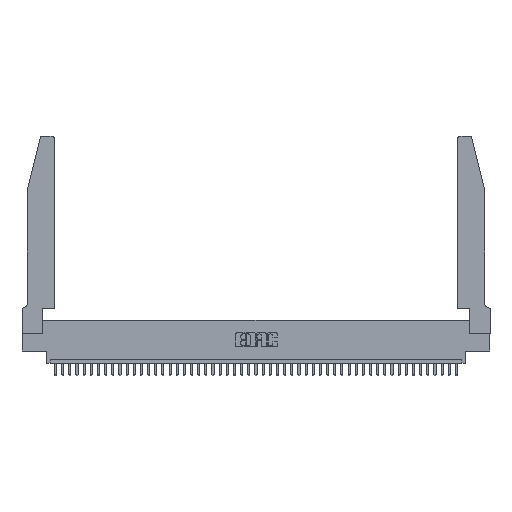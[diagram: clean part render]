
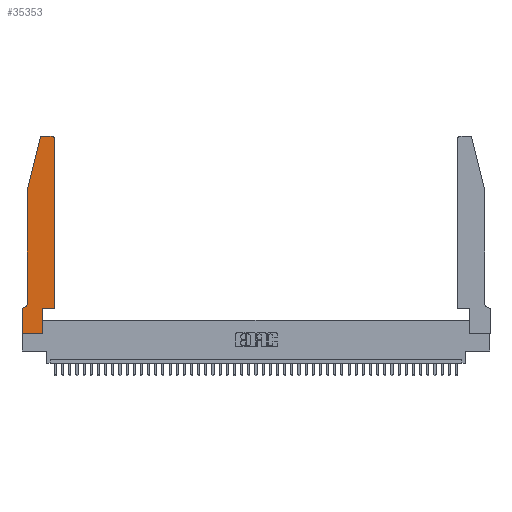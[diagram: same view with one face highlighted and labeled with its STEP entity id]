
A CAD part, top view. The second image highlights one B-rep face of the part: STEP entity #35353.
In plain terms, the highlighted planar face has unit normal (0, 0, 1).
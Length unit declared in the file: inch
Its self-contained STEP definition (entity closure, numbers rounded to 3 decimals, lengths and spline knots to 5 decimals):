
#238 = ORIENTED_EDGE ( 'NONE', *, *, #34138, .T. ) ;
#360 = EDGE_CURVE ( 'NONE', #20974, #18278, #41906, .T. ) ;
#923 = CARTESIAN_POINT ( 'NONE',  ( 0., 0.35, 0.37 ) ) ;
#1006 = CARTESIAN_POINT ( 'NONE',  ( 0., 0., 0.37 ) ) ;
#1175 = CARTESIAN_POINT ( 'NONE',  ( 0.2605, 2.75, 0.37 ) ) ;
#1420 = CARTESIAN_POINT ( 'NONE',  ( 0.2865, 0.35, 0.37 ) ) ;
#1841 = DIRECTION ( 'NONE',  ( 1., 0., 0. ) ) ;
#2367 = ORIENTED_EDGE ( 'NONE', *, *, #9281, .T. ) ;
#2576 = ORIENTED_EDGE ( 'NONE', *, *, #35961, .T. ) ;
#2604 = LINE ( 'NONE', #16483, #27012 ) ;
#2642 = CARTESIAN_POINT ( 'NONE',  ( 0.2865, 0.35, 0.37 ) ) ;
#3133 = DIRECTION ( 'NONE',  ( -1., 0., 0. ) ) ;
#3793 = ORIENTED_EDGE ( 'NONE', *, *, #360, .T. ) ;
#4416 = CARTESIAN_POINT ( 'NONE',  ( 0., 0.35, 0.37 ) ) ;
#4430 = DIRECTION ( 'NONE',  ( -1., 0., 0. ) ) ;
#4469 = ORIENTED_EDGE ( 'NONE', *, *, #27929, .T. ) ;
#4613 = CARTESIAN_POINT ( 'NONE',  ( 0., 0., 0.37 ) ) ;
#4697 = CARTESIAN_POINT ( 'NONE',  ( 0.4505, 0.35, 0.37 ) ) ;
#5005 = VECTOR ( 'NONE', #39588, 39.37008 ) ;
#5119 = CARTESIAN_POINT ( 'NONE',  ( 0.0755, 2., 0.37 ) ) ;
#5654 = CIRCLE ( 'NONE', #28193, 0.07 ) ;
#6397 = VERTEX_POINT ( 'NONE', #923 ) ;
#6874 = CARTESIAN_POINT ( 'NONE',  ( 0.2865, 0., 0.37 ) ) ;
#7835 = DIRECTION ( 'NONE',  ( 1., 0., 0. ) ) ;
#7964 = CARTESIAN_POINT ( 'NONE',  ( 0.0755, 2., 0.37 ) ) ;
#8586 = CARTESIAN_POINT ( 'NONE',  ( 0.4505, 0.35, 0.37 ) ) ;
#8760 = DIRECTION ( 'NONE',  ( 0., -1., 0. ) ) ;
#8840 = VECTOR ( 'NONE', #31406, 39.37008 ) ;
#9281 = EDGE_CURVE ( 'NONE', #23190, #41723, #2604, .T. ) ;
#10288 = ORIENTED_EDGE ( 'NONE', *, *, #40681, .T. ) ;
#10289 = DIRECTION ( 'NONE',  ( 0., 0., -1. ) ) ;
#10429 = CARTESIAN_POINT ( 'NONE',  ( 0.0055, 0.35, 0.37 ) ) ;
#10708 = EDGE_CURVE ( 'NONE', #18545, #32068, #42664, .T. ) ;
#10870 = EDGE_LOOP ( 'NONE', ( #25794, #3793, #2576, #2367, #238, #40316, #20982, #4469, #16432, #30273, #12661, #10288 ) ) ;
#10888 = EDGE_CURVE ( 'NONE', #21116, #18545, #12234, .T. ) ;
#11809 = DIRECTION ( 'NONE',  ( -0.239, -0.971, 0. ) ) ;
#11862 = PLANE ( 'NONE',  #31098 ) ;
#12083 = VECTOR ( 'NONE', #36885, 39.37008 ) ;
#12234 = LINE ( 'NONE', #1420, #22256 ) ;
#12385 = DIRECTION ( 'NONE',  ( 1., 0., 0. ) ) ;
#12661 = ORIENTED_EDGE ( 'NONE', *, *, #30907, .T. ) ;
#13523 = CARTESIAN_POINT ( 'NONE',  ( 0.0055, 0.42, 0.37 ) ) ;
#15779 = DIRECTION ( 'NONE',  ( 0., 0., 1. ) ) ;
#16129 = LINE ( 'NONE', #1175, #27207 ) ;
#16432 = ORIENTED_EDGE ( 'NONE', *, *, #10888, .T. ) ;
#16483 = CARTESIAN_POINT ( 'NONE',  ( 0.0755, 2., 0.37 ) ) ;
#16660 = LINE ( 'NONE', #1006, #5005 ) ;
#16927 = EDGE_CURVE ( 'NONE', #45058, #6397, #34087, .T. ) ;
#17163 = LINE ( 'NONE', #8586, #8840 ) ;
#18278 = VERTEX_POINT ( 'NONE', #44813 ) ;
#18534 = DIRECTION ( 'NONE',  ( 0., 0., 1. ) ) ;
#18545 = VERTEX_POINT ( 'NONE', #2642 ) ;
#20974 = VERTEX_POINT ( 'NONE', #28274 ) ;
#20982 = ORIENTED_EDGE ( 'NONE', *, *, #26684, .T. ) ;
#21116 = VERTEX_POINT ( 'NONE', #6874 ) ;
#22256 = VECTOR ( 'NONE', #33385, 39.37008 ) ;
#23190 = VERTEX_POINT ( 'NONE', #7964 ) ;
#23413 = AXIS2_PLACEMENT_3D ( 'NONE', #28247, #35282, #38821 ) ;
#24199 = CARTESIAN_POINT ( 'NONE',  ( 0.0755, 0.35, 0.37 ) ) ;
#25794 = ORIENTED_EDGE ( 'NONE', *, *, #38031, .T. ) ;
#26684 = EDGE_CURVE ( 'NONE', #6397, #29456, #16660, .T. ) ;
#27012 = VECTOR ( 'NONE', #8760, 39.37008 ) ;
#27207 = VECTOR ( 'NONE', #4430, 39.37008 ) ;
#27929 = EDGE_CURVE ( 'NONE', #29456, #21116, #40213, .T. ) ;
#28193 = AXIS2_PLACEMENT_3D ( 'NONE', #13523, #10289, #3133 ) ;
#28247 = CARTESIAN_POINT ( 'NONE',  ( 0.284, 2.72, 0.37 ) ) ;
#28274 = CARTESIAN_POINT ( 'NONE',  ( 0.284, 2.75, 0.37 ) ) ;
#28393 = CARTESIAN_POINT ( 'NONE',  ( 0.4505, 2.72, 0.37 ) ) ;
#29456 = VERTEX_POINT ( 'NONE', #43304 ) ;
#29823 = CARTESIAN_POINT ( 'NONE',  ( 0.4505, 0.35, 0.37 ) ) ;
#30273 = ORIENTED_EDGE ( 'NONE', *, *, #10708, .T. ) ;
#30513 = VERTEX_POINT ( 'NONE', #28393 ) ;
#30907 = EDGE_CURVE ( 'NONE', #32068, #30513, #17163, .T. ) ;
#31098 = AXIS2_PLACEMENT_3D ( 'NONE', #4416, #18534, #7835 ) ;
#31406 = DIRECTION ( 'NONE',  ( 0., 1., 0. ) ) ;
#32068 = VERTEX_POINT ( 'NONE', #4697 ) ;
#33385 = DIRECTION ( 'NONE',  ( 0., 1., 0. ) ) ;
#33811 = CIRCLE ( 'NONE', #43741, 0.03 ) ;
#34087 = LINE ( 'NONE', #24199, #39618 ) ;
#34138 = EDGE_CURVE ( 'NONE', #41723, #45058, #5654, .T. ) ;
#34336 = VECTOR ( 'NONE', #12385, 39.37008 ) ;
#35140 = DIRECTION ( 'NONE',  ( -1., 0., 0. ) ) ;
#35282 = DIRECTION ( 'NONE',  ( 0., 0., 1. ) ) ;
#35353 = ADVANCED_FACE ( 'NONE', ( #40342 ), #11862, .T. ) ;
#35558 = LINE ( 'NONE', #5119, #43942 ) ;
#35961 = EDGE_CURVE ( 'NONE', #18278, #23190, #35558, .T. ) ;
#36454 = CARTESIAN_POINT ( 'NONE',  ( 0.0755, 0.42, 0.37 ) ) ;
#36885 = DIRECTION ( 'NONE',  ( 1., 0., 0. ) ) ;
#38031 = EDGE_CURVE ( 'NONE', #42253, #20974, #16129, .T. ) ;
#38821 = DIRECTION ( 'NONE',  ( 1., 0., 0. ) ) ;
#39186 = CARTESIAN_POINT ( 'NONE',  ( 0.4205, 2.75, 0.37 ) ) ;
#39588 = DIRECTION ( 'NONE',  ( 0., -1., 0. ) ) ;
#39618 = VECTOR ( 'NONE', #35140, 39.37008 ) ;
#40213 = LINE ( 'NONE', #4613, #12083 ) ;
#40316 = ORIENTED_EDGE ( 'NONE', *, *, #16927, .T. ) ;
#40342 = FACE_OUTER_BOUND ( 'NONE', #10870, .T. ) ;
#40681 = EDGE_CURVE ( 'NONE', #30513, #42253, #33811, .T. ) ;
#41723 = VERTEX_POINT ( 'NONE', #36454 ) ;
#41906 = CIRCLE ( 'NONE', #23413, 0.03 ) ;
#42253 = VERTEX_POINT ( 'NONE', #39186 ) ;
#42664 = LINE ( 'NONE', #29823, #34336 ) ;
#43304 = CARTESIAN_POINT ( 'NONE',  ( 0., 0., 0.37 ) ) ;
#43741 = AXIS2_PLACEMENT_3D ( 'NONE', #44703, #15779, #1841 ) ;
#43942 = VECTOR ( 'NONE', #11809, 39.37008 ) ;
#44703 = CARTESIAN_POINT ( 'NONE',  ( 0.4205, 2.72, 0.37 ) ) ;
#44813 = CARTESIAN_POINT ( 'NONE',  ( 0.25487, 2.72718, 0.37 ) ) ;
#45058 = VERTEX_POINT ( 'NONE', #10429 ) ;
